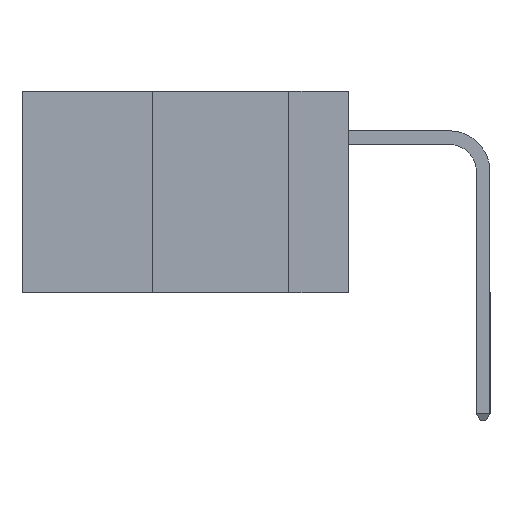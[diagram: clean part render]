
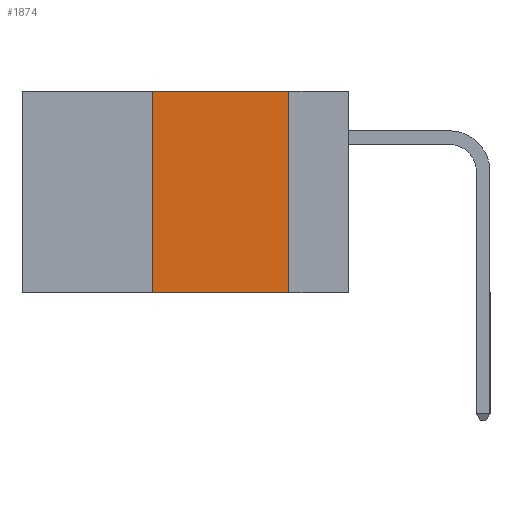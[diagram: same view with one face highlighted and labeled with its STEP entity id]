
A CAD part, left-side view. The second image highlights one B-rep face of the part: STEP entity #1874.
In plain terms, the highlighted planar face has unit normal (-1, 0, 0).
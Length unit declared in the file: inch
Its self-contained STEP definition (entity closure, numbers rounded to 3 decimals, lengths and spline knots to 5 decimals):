
#443 = EDGE_LOOP ( 'NONE', ( #8962, #7649, #2517, #7837 ) ) ;
#516 = CARTESIAN_POINT ( 'NONE',  ( 0., 0.36, 0. ) ) ;
#569 = DIRECTION ( 'NONE',  ( 0., -1., 0. ) ) ;
#679 = VECTOR ( 'NONE', #5679, 39.37008 ) ;
#885 = CARTESIAN_POINT ( 'NONE',  ( 0., 0.6, -0.37 ) ) ;
#937 = VERTEX_POINT ( 'NONE', #516 ) ;
#971 = CARTESIAN_POINT ( 'NONE',  ( 0., 0.11, 0. ) ) ;
#1052 = VECTOR ( 'NONE', #569, 39.37008 ) ;
#1212 = DIRECTION ( 'NONE',  ( 0., 0., -1. ) ) ;
#1286 = DIRECTION ( 'NONE',  ( 1., 0., 0. ) ) ;
#1345 = CARTESIAN_POINT ( 'NONE',  ( 0., 0.6, 0. ) ) ;
#1430 = CARTESIAN_POINT ( 'NONE',  ( 0., 0.11, -0.37 ) ) ;
#1874 = ADVANCED_FACE ( 'NONE', ( #2833 ), #3852, .F. ) ;
#2517 = ORIENTED_EDGE ( 'NONE', *, *, #6975, .F. ) ;
#2610 = CARTESIAN_POINT ( 'NONE',  ( 0., 0.6, 0. ) ) ;
#2833 = FACE_OUTER_BOUND ( 'NONE', #443, .T. ) ;
#2899 = AXIS2_PLACEMENT_3D ( 'NONE', #1345, #1286, #1212 ) ;
#3182 = LINE ( 'NONE', #2610, #6574 ) ;
#3250 = VERTEX_POINT ( 'NONE', #1430 ) ;
#3379 = DIRECTION ( 'NONE',  ( 0., -1., 0. ) ) ;
#3852 = PLANE ( 'NONE',  #2899 ) ;
#3860 = LINE ( 'NONE', #5970, #8853 ) ;
#4090 = EDGE_CURVE ( 'NONE', #5500, #3250, #8138, .T. ) ;
#5500 = VERTEX_POINT ( 'NONE', #971 ) ;
#5652 = VERTEX_POINT ( 'NONE', #8942 ) ;
#5679 = DIRECTION ( 'NONE',  ( 0., 0., -1. ) ) ;
#5969 = DIRECTION ( 'NONE',  ( 0., 0., 1. ) ) ;
#5970 = CARTESIAN_POINT ( 'NONE',  ( 0., 0.36, 0. ) ) ;
#6286 = EDGE_CURVE ( 'NONE', #5652, #3250, #6406, .T. ) ;
#6406 = LINE ( 'NONE', #885, #1052 ) ;
#6574 = VECTOR ( 'NONE', #3379, 39.37008 ) ;
#6589 = CARTESIAN_POINT ( 'NONE',  ( 0., 0.11, 0. ) ) ;
#6975 = EDGE_CURVE ( 'NONE', #5652, #937, #3860, .T. ) ;
#7649 = ORIENTED_EDGE ( 'NONE', *, *, #8590, .F. ) ;
#7837 = ORIENTED_EDGE ( 'NONE', *, *, #6286, .T. ) ;
#8138 = LINE ( 'NONE', #6589, #679 ) ;
#8590 = EDGE_CURVE ( 'NONE', #937, #5500, #3182, .T. ) ;
#8853 = VECTOR ( 'NONE', #5969, 39.37008 ) ;
#8942 = CARTESIAN_POINT ( 'NONE',  ( 0., 0.36, -0.37 ) ) ;
#8962 = ORIENTED_EDGE ( 'NONE', *, *, #4090, .F. ) ;
